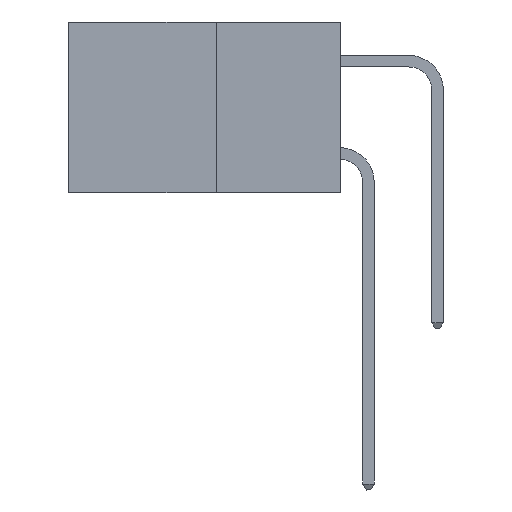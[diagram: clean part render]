
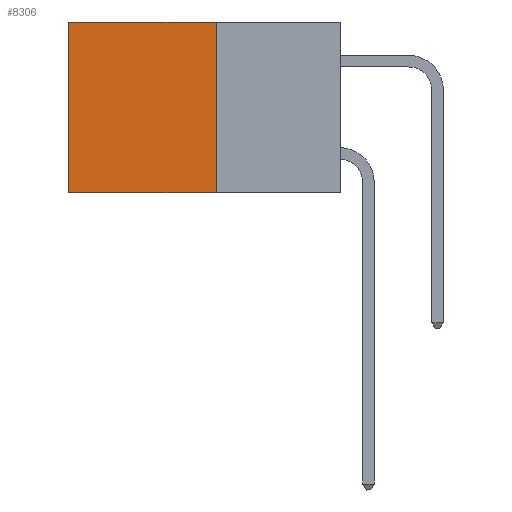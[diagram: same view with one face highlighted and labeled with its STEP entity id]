
A CAD part, left-side view. The second image highlights one B-rep face of the part: STEP entity #8306.
In plain terms, the highlighted planar face has unit normal (-1, 0, 0).
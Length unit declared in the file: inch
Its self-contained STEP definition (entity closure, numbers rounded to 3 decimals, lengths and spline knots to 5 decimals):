
#150 = AXIS2_PLACEMENT_3D ( 'NONE', #5883, #19772, #9475 ) ;
#1461 = LINE ( 'NONE', #16067, #5669 ) ;
#2073 = LINE ( 'NONE', #14894, #9918 ) ;
#3130 = EDGE_CURVE ( 'NONE', #3974, #7576, #1461, .T. ) ;
#3591 = CARTESIAN_POINT ( 'NONE',  ( 0.277, 0.27, -0.37 ) ) ;
#3623 = ORIENTED_EDGE ( 'NONE', *, *, #21498, .T. ) ;
#3910 = VERTEX_POINT ( 'NONE', #15162 ) ;
#3974 = VERTEX_POINT ( 'NONE', #7197 ) ;
#4419 = CARTESIAN_POINT ( 'NONE',  ( 0.277, 0.59, 0. ) ) ;
#5095 = DIRECTION ( 'NONE',  ( 0., 0., -1. ) ) ;
#5669 = VECTOR ( 'NONE', #20759, 39.37008 ) ;
#5778 = VECTOR ( 'NONE', #17619, 39.37008 ) ;
#5883 = CARTESIAN_POINT ( 'NONE',  ( 0.277, 0.27, -0.37 ) ) ;
#6109 = DIRECTION ( 'NONE',  ( 0., 1., 0. ) ) ;
#6902 = LINE ( 'NONE', #3591, #5778 ) ;
#7197 = CARTESIAN_POINT ( 'NONE',  ( 0.277, 0.27, 0. ) ) ;
#7576 = VERTEX_POINT ( 'NONE', #4419 ) ;
#8306 = ADVANCED_FACE ( 'NONE', ( #13593 ), #14673, .F. ) ;
#9475 = DIRECTION ( 'NONE',  ( 0., 0., -1. ) ) ;
#9918 = VECTOR ( 'NONE', #6109, 39.37008 ) ;
#10111 = ORIENTED_EDGE ( 'NONE', *, *, #11223, .F. ) ;
#11013 = VERTEX_POINT ( 'NONE', #13078 ) ;
#11223 = EDGE_CURVE ( 'NONE', #3910, #11013, #2073, .T. ) ;
#11384 = ORIENTED_EDGE ( 'NONE', *, *, #3130, .T. ) ;
#12298 = EDGE_CURVE ( 'NONE', #3974, #3910, #6902, .T. ) ;
#13078 = CARTESIAN_POINT ( 'NONE',  ( 0.277, 0.59, -0.37 ) ) ;
#13089 = VECTOR ( 'NONE', #5095, 39.37008 ) ;
#13593 = FACE_OUTER_BOUND ( 'NONE', #20008, .T. ) ;
#14673 = PLANE ( 'NONE',  #150 ) ;
#14894 = CARTESIAN_POINT ( 'NONE',  ( 0.277, 0.27, -0.37 ) ) ;
#15162 = CARTESIAN_POINT ( 'NONE',  ( 0.277, 0.27, -0.37 ) ) ;
#15648 = CARTESIAN_POINT ( 'NONE',  ( 0.277, 0.59, -0.37 ) ) ;
#16067 = CARTESIAN_POINT ( 'NONE',  ( 0.277, 0.27, 0. ) ) ;
#16829 = ORIENTED_EDGE ( 'NONE', *, *, #12298, .F. ) ;
#17619 = DIRECTION ( 'NONE',  ( 0., 0., -1. ) ) ;
#17634 = LINE ( 'NONE', #15648, #13089 ) ;
#19772 = DIRECTION ( 'NONE',  ( 1., 0., 0. ) ) ;
#20008 = EDGE_LOOP ( 'NONE', ( #3623, #10111, #16829, #11384 ) ) ;
#20759 = DIRECTION ( 'NONE',  ( 0., 1., 0. ) ) ;
#21498 = EDGE_CURVE ( 'NONE', #7576, #11013, #17634, .T. ) ;
